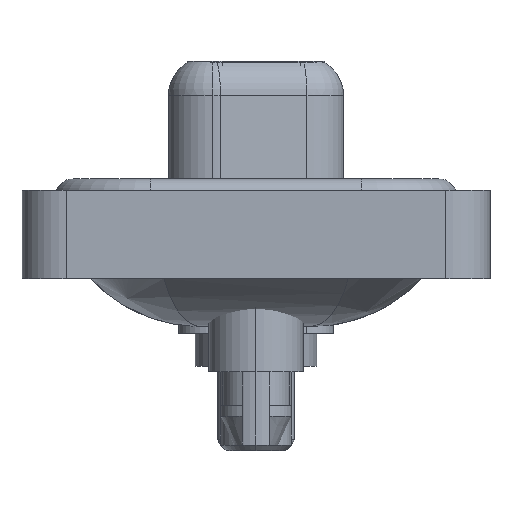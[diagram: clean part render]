
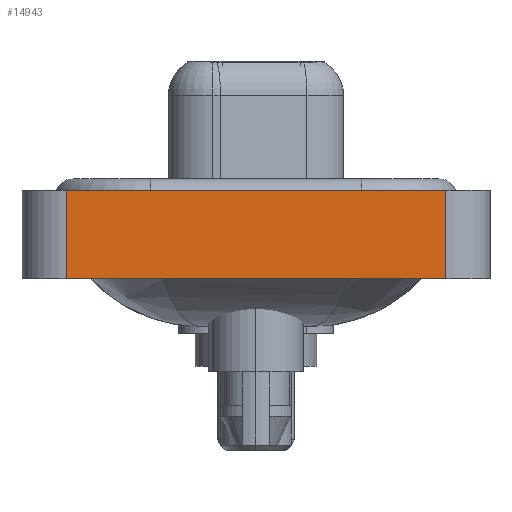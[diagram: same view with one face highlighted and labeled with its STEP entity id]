
A CAD part, left-side view. The second image highlights one B-rep face of the part: STEP entity #14943.
In plain terms, the highlighted planar face has unit normal (-1, 0, 0).
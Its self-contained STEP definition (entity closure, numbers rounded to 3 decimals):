
#836 = CARTESIAN_POINT ( 'NONE',  ( -7.3, -8.55, -3.6 ) ) ;
#856 = VERTEX_POINT ( 'NONE', #9902 ) ;
#1732 = ORIENTED_EDGE ( 'NONE', *, *, #15474, .F. ) ;
#2381 = PLANE ( 'NONE',  #5017 ) ;
#2980 = ORIENTED_EDGE ( 'NONE', *, *, #8258, .F. ) ;
#3183 = LINE ( 'NONE', #6846, #17368 ) ;
#3921 = EDGE_CURVE ( 'NONE', #6883, #9975, #7164, .T. ) ;
#4903 = VERTEX_POINT ( 'NONE', #14552 ) ;
#5017 = AXIS2_PLACEMENT_3D ( 'NONE', #836, #14404, #21246 ) ;
#5587 = DIRECTION ( 'NONE',  ( 0., 0., 1. ) ) ;
#6468 = VECTOR ( 'NONE', #8300, 1000. ) ;
#6846 = CARTESIAN_POINT ( 'NONE',  ( -7.3, -8.55, 0.4 ) ) ;
#6883 = VERTEX_POINT ( 'NONE', #19310 ) ;
#6951 = DIRECTION ( 'NONE',  ( 0., -1., 0. ) ) ;
#7164 = LINE ( 'NONE', #17613, #8257 ) ;
#8257 = VECTOR ( 'NONE', #9137, 1000. ) ;
#8258 = EDGE_CURVE ( 'NONE', #856, #4903, #3183, .T. ) ;
#8300 = DIRECTION ( 'NONE',  ( 0., 0., 1. ) ) ;
#9121 = LINE ( 'NONE', #14380, #19573 ) ;
#9137 = DIRECTION ( 'NONE',  ( 0., -1., 0. ) ) ;
#9553 = EDGE_CURVE ( 'NONE', #9975, #4903, #13548, .T. ) ;
#9888 = EDGE_LOOP ( 'NONE', ( #21031, #2980, #1732, #15118 ) ) ;
#9902 = CARTESIAN_POINT ( 'NONE',  ( -7.3, 8.55, 0.4 ) ) ;
#9975 = VERTEX_POINT ( 'NONE', #16277 ) ;
#13548 = LINE ( 'NONE', #15201, #6468 ) ;
#14380 = CARTESIAN_POINT ( 'NONE',  ( -7.3, 8.55, -3.6 ) ) ;
#14404 = DIRECTION ( 'NONE',  ( -1., 0., 0. ) ) ;
#14552 = CARTESIAN_POINT ( 'NONE',  ( -7.3, -8.55, 0.4 ) ) ;
#14943 = ADVANCED_FACE ( 'NONE', ( #20818 ), #2381, .T. ) ;
#15118 = ORIENTED_EDGE ( 'NONE', *, *, #3921, .T. ) ;
#15201 = CARTESIAN_POINT ( 'NONE',  ( -7.3, -8.55, -3.6 ) ) ;
#15474 = EDGE_CURVE ( 'NONE', #6883, #856, #9121, .T. ) ;
#16277 = CARTESIAN_POINT ( 'NONE',  ( -7.3, -8.55, -3.6 ) ) ;
#17368 = VECTOR ( 'NONE', #6951, 1000. ) ;
#17613 = CARTESIAN_POINT ( 'NONE',  ( -7.3, -8.55, -3.6 ) ) ;
#19310 = CARTESIAN_POINT ( 'NONE',  ( -7.3, 8.55, -3.6 ) ) ;
#19573 = VECTOR ( 'NONE', #5587, 1000. ) ;
#20818 = FACE_OUTER_BOUND ( 'NONE', #9888, .T. ) ;
#21031 = ORIENTED_EDGE ( 'NONE', *, *, #9553, .T. ) ;
#21246 = DIRECTION ( 'NONE',  ( 0., 0., 1. ) ) ;
